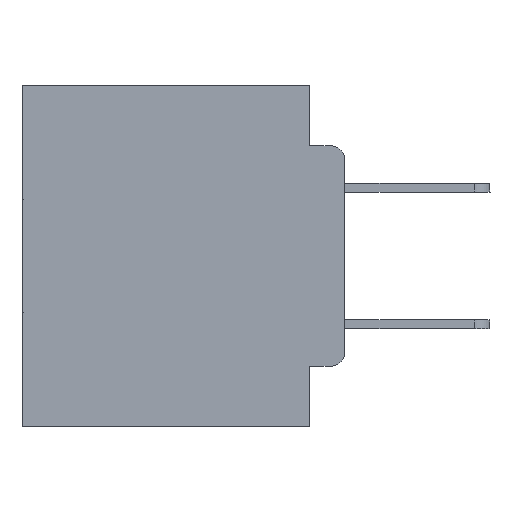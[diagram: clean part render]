
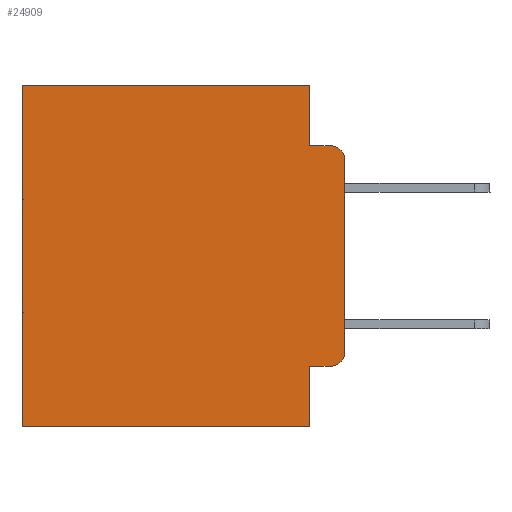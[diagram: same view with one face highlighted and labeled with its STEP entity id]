
A CAD part, left-side view. The second image highlights one B-rep face of the part: STEP entity #24909.
In plain terms, the highlighted planar face has unit normal (-1, 0, 0).
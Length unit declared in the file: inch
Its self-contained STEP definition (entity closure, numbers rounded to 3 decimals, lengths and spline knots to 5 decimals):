
#1788 = CARTESIAN_POINT ( 'NONE',  ( 0.298, 0., -0.5 ) ) ;
#2642 = LINE ( 'NONE', #23790, #7314 ) ;
#2921 = VERTEX_POINT ( 'NONE', #14920 ) ;
#3450 = VECTOR ( 'NONE', #17603, 39.37008 ) ;
#4949 = CARTESIAN_POINT ( 'NONE',  ( 0.298, 0.473, -0.5 ) ) ;
#5330 = CARTESIAN_POINT ( 'NONE',  ( 0.298, 0.051, -0.5 ) ) ;
#5518 = VECTOR ( 'NONE', #13235, 39.37008 ) ;
#6068 = EDGE_CURVE ( 'NONE', #17629, #19013, #12333, .T. ) ;
#6445 = VERTEX_POINT ( 'NONE', #28655 ) ;
#6663 = DIRECTION ( 'NONE',  ( -1., 0., 0. ) ) ;
#6907 = EDGE_CURVE ( 'NONE', #6445, #9416, #2642, .T. ) ;
#7314 = VECTOR ( 'NONE', #18966, 39.37008 ) ;
#8362 = VECTOR ( 'NONE', #8929, 39.37008 ) ;
#8712 = LINE ( 'NONE', #25604, #19679 ) ;
#8863 = EDGE_CURVE ( 'NONE', #18189, #21127, #11263, .T. ) ;
#8911 = AXIS2_PLACEMENT_3D ( 'NONE', #30564, #18707, #12394 ) ;
#8929 = DIRECTION ( 'NONE',  ( 0., -1., 0. ) ) ;
#9416 = VERTEX_POINT ( 'NONE', #4949 ) ;
#9431 = VERTEX_POINT ( 'NONE', #21386 ) ;
#9597 = ORIENTED_EDGE ( 'NONE', *, *, #19023, .T. ) ;
#9773 = EDGE_CURVE ( 'NONE', #17629, #21127, #20404, .T. ) ;
#9793 = VECTOR ( 'NONE', #26404, 39.37008 ) ;
#9887 = CARTESIAN_POINT ( 'NONE',  ( 0.298, 0., 0. ) ) ;
#11263 = LINE ( 'NONE', #30332, #8362 ) ;
#12333 = LINE ( 'NONE', #26548, #9793 ) ;
#12394 = DIRECTION ( 'NONE',  ( 0., 0., -1. ) ) ;
#13235 = DIRECTION ( 'NONE',  ( 0., 1., 0. ) ) ;
#14413 = AXIS2_PLACEMENT_3D ( 'NONE', #26366, #16658, #19328 ) ;
#14920 = CARTESIAN_POINT ( 'NONE',  ( 0.298, 0.02, -0.4115 ) ) ;
#16373 = CARTESIAN_POINT ( 'NONE',  ( 0.298, 0., -0.3915 ) ) ;
#16658 = DIRECTION ( 'NONE',  ( 1., 0., 0. ) ) ;
#16896 = ORIENTED_EDGE ( 'NONE', *, *, #28390, .T. ) ;
#17135 = CARTESIAN_POINT ( 'NONE',  ( 0.298, 0.051, 0. ) ) ;
#17455 = LINE ( 'NONE', #17135, #3450 ) ;
#17603 = DIRECTION ( 'NONE',  ( 0., 0., -1. ) ) ;
#17629 = VERTEX_POINT ( 'NONE', #26092 ) ;
#18008 = ORIENTED_EDGE ( 'NONE', *, *, #28899, .F. ) ;
#18189 = VERTEX_POINT ( 'NONE', #19142 ) ;
#18608 = PLANE ( 'NONE',  #14413 ) ;
#18707 = DIRECTION ( 'NONE',  ( -1., 0., 0. ) ) ;
#18834 = VERTEX_POINT ( 'NONE', #19689 ) ;
#18966 = DIRECTION ( 'NONE',  ( 0., 0., -1. ) ) ;
#19013 = VERTEX_POINT ( 'NONE', #16373 ) ;
#19023 = EDGE_CURVE ( 'NONE', #9431, #2921, #8712, .T. ) ;
#19142 = CARTESIAN_POINT ( 'NONE',  ( 0.298, 0.051, -0.0885 ) ) ;
#19144 = VECTOR ( 'NONE', #19439, 39.37008 ) ;
#19328 = DIRECTION ( 'NONE',  ( 0., 0., -1. ) ) ;
#19439 = DIRECTION ( 'NONE',  ( 0., 1., 0. ) ) ;
#19679 = VECTOR ( 'NONE', #29972, 39.37008 ) ;
#19689 = CARTESIAN_POINT ( 'NONE',  ( 0.298, 0.051, 0. ) ) ;
#20404 = CIRCLE ( 'NONE', #8911, 0.02 ) ;
#20438 = DIRECTION ( 'NONE',  ( 0., 0., -1. ) ) ;
#20744 = CARTESIAN_POINT ( 'NONE',  ( 0.298, 0.02, -0.3915 ) ) ;
#21123 = CARTESIAN_POINT ( 'NONE',  ( 0.298, 0.02, -0.0885 ) ) ;
#21127 = VERTEX_POINT ( 'NONE', #21123 ) ;
#21386 = CARTESIAN_POINT ( 'NONE',  ( 0.298, 0.051, -0.4115 ) ) ;
#21757 = LINE ( 'NONE', #9887, #19144 ) ;
#23009 = ORIENTED_EDGE ( 'NONE', *, *, #28859, .T. ) ;
#23229 = LINE ( 'NONE', #1788, #5518 ) ;
#23380 = ORIENTED_EDGE ( 'NONE', *, *, #6068, .F. ) ;
#23790 = CARTESIAN_POINT ( 'NONE',  ( 0.298, 0.473, 0. ) ) ;
#24087 = ORIENTED_EDGE ( 'NONE', *, *, #27606, .F. ) ;
#24909 = ADVANCED_FACE ( 'NONE', ( #26655 ), #18608, .F. ) ;
#25417 = ORIENTED_EDGE ( 'NONE', *, *, #26111, .F. ) ;
#25604 = CARTESIAN_POINT ( 'NONE',  ( 0.298, 0.051, -0.4115 ) ) ;
#26092 = CARTESIAN_POINT ( 'NONE',  ( 0.298, 0., -0.1085 ) ) ;
#26111 = EDGE_CURVE ( 'NONE', #9431, #29886, #17455, .T. ) ;
#26366 = CARTESIAN_POINT ( 'NONE',  ( 0.298, 0., 0. ) ) ;
#26404 = DIRECTION ( 'NONE',  ( 0., 0., -1. ) ) ;
#26548 = CARTESIAN_POINT ( 'NONE',  ( 0.298, 0., 0. ) ) ;
#26622 = CIRCLE ( 'NONE', #30624, 0.02 ) ;
#26655 = FACE_OUTER_BOUND ( 'NONE', #29378, .T. ) ;
#27582 = ORIENTED_EDGE ( 'NONE', *, *, #8863, .F. ) ;
#27606 = EDGE_CURVE ( 'NONE', #29886, #9416, #23229, .T. ) ;
#27607 = DIRECTION ( 'NONE',  ( 0., 0., -1. ) ) ;
#27631 = VECTOR ( 'NONE', #27607, 39.37008 ) ;
#28390 = EDGE_CURVE ( 'NONE', #18834, #6445, #21757, .T. ) ;
#28655 = CARTESIAN_POINT ( 'NONE',  ( 0.298, 0.473, 0. ) ) ;
#28839 = ORIENTED_EDGE ( 'NONE', *, *, #6907, .T. ) ;
#28859 = EDGE_CURVE ( 'NONE', #2921, #19013, #26622, .T. ) ;
#28899 = EDGE_CURVE ( 'NONE', #18834, #18189, #30104, .T. ) ;
#29378 = EDGE_LOOP ( 'NONE', ( #23380, #29593, #27582, #18008, #16896, #28839, #24087, #25417, #9597, #23009 ) ) ;
#29593 = ORIENTED_EDGE ( 'NONE', *, *, #9773, .T. ) ;
#29886 = VERTEX_POINT ( 'NONE', #5330 ) ;
#29972 = DIRECTION ( 'NONE',  ( 0., -1., 0. ) ) ;
#30104 = LINE ( 'NONE', #30264, #27631 ) ;
#30264 = CARTESIAN_POINT ( 'NONE',  ( 0.298, 0.051, 0. ) ) ;
#30332 = CARTESIAN_POINT ( 'NONE',  ( 0.298, 0.051, -0.0885 ) ) ;
#30564 = CARTESIAN_POINT ( 'NONE',  ( 0.298, 0.02, -0.1085 ) ) ;
#30624 = AXIS2_PLACEMENT_3D ( 'NONE', #20744, #6663, #20438 ) ;
